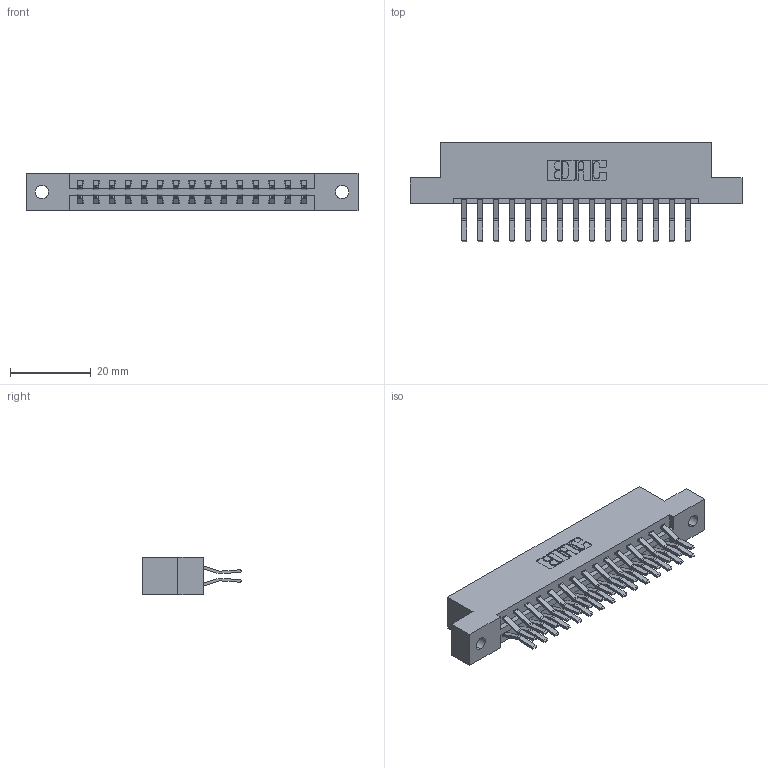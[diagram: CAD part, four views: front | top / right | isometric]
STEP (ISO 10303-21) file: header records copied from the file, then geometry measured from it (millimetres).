
FILE_DESCRIPTION (( 'STEP AP203' ), '1' );
FILE_NAME ('337-030-560-202.STEP', '2018-08-07T02:35:42', ( '' ), ( '' ), 'SwSTEP 2.0', 'SolidWorks 2016', '' );
FILE_SCHEMA (( 'CONFIG_CONTROL_DESIGN' ));
Length unit declared in the file: inch
Products named in the file (3): 337-030-560-202; 337 Part_Flush Mounting Lugs - 0.128 Dia; 345-292-001_560 Tail
Assembly tree (31 placements, depth 2):
  337-030-560-202
    337 Part_Flush Mounting Lugs - 0.128 Dia
    345-292-001_560 Tail  x30
Bounding box: 82.45 x 24.78 x 9.4 mm (x, y, z)
Volume: 8489.6 mm3; surface area: 9631.7 mm2
Topology: 31 solids, 31 shells, 1794 faces, 5321 edges, 3506 vertices
Faces by surface type: plane 1210, cylinder 584
Entity records: 15213 total; most frequent: CARTESIAN_POINT 2586, ORIENTED_EDGE 2522, DIRECTION 2253, EDGE_CURVE 1261, LINE 1129, VECTOR 1129, VERTEX_POINT 838, AXIS2_PLACEMENT_3D 562
